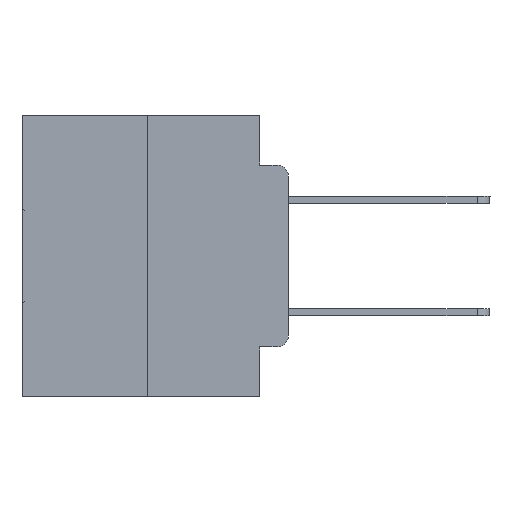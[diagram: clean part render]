
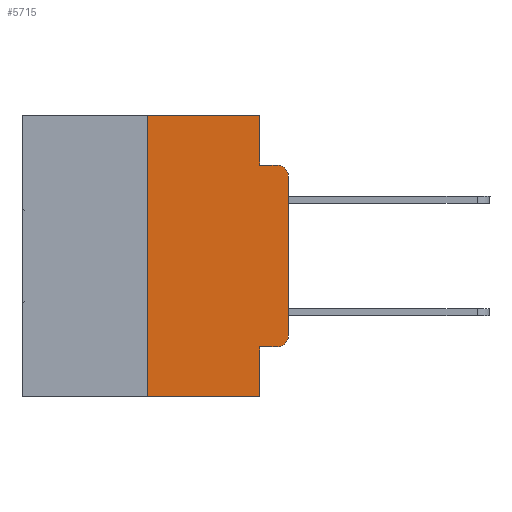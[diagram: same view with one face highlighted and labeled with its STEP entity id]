
A CAD part, left-side view. The second image highlights one B-rep face of the part: STEP entity #5715.
In plain terms, the highlighted planar face has unit normal (-1, 0, 0).
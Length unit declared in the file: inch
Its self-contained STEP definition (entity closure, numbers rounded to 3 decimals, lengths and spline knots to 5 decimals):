
#12 = CARTESIAN_POINT ( 'NONE',  ( 0., 0.473, 0. ) ) ;
#261 = DIRECTION ( 'NONE',  ( 0., 0., -1. ) ) ;
#588 = CARTESIAN_POINT ( 'NONE',  ( 0., 0.02, -0.4115 ) ) ;
#1628 = PLANE ( 'NONE',  #4359 ) ;
#1632 = VERTEX_POINT ( 'NONE', #25571 ) ;
#2724 = VERTEX_POINT ( 'NONE', #16034 ) ;
#2810 = DIRECTION ( 'NONE',  ( -1., 0., 0. ) ) ;
#2978 = VERTEX_POINT ( 'NONE', #13613 ) ;
#3364 = ORIENTED_EDGE ( 'NONE', *, *, #14036, .T. ) ;
#4012 = CARTESIAN_POINT ( 'NONE',  ( 0., 0.473, 0. ) ) ;
#4062 = CARTESIAN_POINT ( 'NONE',  ( 0., 0.051, -0.5 ) ) ;
#4359 = AXIS2_PLACEMENT_3D ( 'NONE', #4012, #8767, #25254 ) ;
#4379 = VECTOR ( 'NONE', #29222, 39.37008 ) ;
#4464 = CARTESIAN_POINT ( 'NONE',  ( 0., 0.051, -0.0885 ) ) ;
#4652 = LINE ( 'NONE', #28440, #22053 ) ;
#4831 = ORIENTED_EDGE ( 'NONE', *, *, #28798, .T. ) ;
#5137 = CIRCLE ( 'NONE', #23619, 0.02 ) ;
#5185 = ORIENTED_EDGE ( 'NONE', *, *, #20552, .T. ) ;
#5715 = ADVANCED_FACE ( 'NONE', ( #9387 ), #1628, .F. ) ;
#6418 = VECTOR ( 'NONE', #9989, 39.37008 ) ;
#7110 = CARTESIAN_POINT ( 'NONE',  ( 0., 0.051, 0. ) ) ;
#7713 = LINE ( 'NONE', #4464, #18872 ) ;
#7816 = EDGE_CURVE ( 'NONE', #29315, #2978, #10740, .T. ) ;
#8767 = DIRECTION ( 'NONE',  ( 1., 0., 0. ) ) ;
#8887 = CARTESIAN_POINT ( 'NONE',  ( 0., 0.02, -0.0885 ) ) ;
#9387 = FACE_OUTER_BOUND ( 'NONE', #10035, .T. ) ;
#9423 = EDGE_CURVE ( 'NONE', #18129, #1632, #4652, .T. ) ;
#9897 = EDGE_CURVE ( 'NONE', #2978, #18129, #11405, .T. ) ;
#9989 = DIRECTION ( 'NONE',  ( 0., -1., 0. ) ) ;
#10035 = EDGE_LOOP ( 'NONE', ( #22578, #5185, #17795, #25488, #26896, #21500, #3364, #22965, #4831, #17447 ) ) ;
#10661 = VECTOR ( 'NONE', #25966, 39.37008 ) ;
#10735 = CARTESIAN_POINT ( 'NONE',  ( 0., 0.02, -0.1085 ) ) ;
#10740 = LINE ( 'NONE', #12974, #4379 ) ;
#10758 = CARTESIAN_POINT ( 'NONE',  ( 0., 0., 0. ) ) ;
#10929 = VERTEX_POINT ( 'NONE', #4062 ) ;
#11058 = EDGE_CURVE ( 'NONE', #1632, #17957, #7713, .T. ) ;
#11405 = LINE ( 'NONE', #12, #10661 ) ;
#12974 = CARTESIAN_POINT ( 'NONE',  ( 0., 0.25, 0. ) ) ;
#13109 = DIRECTION ( 'NONE',  ( 0., 0., -1. ) ) ;
#13494 = LINE ( 'NONE', #26385, #6418 ) ;
#13613 = CARTESIAN_POINT ( 'NONE',  ( 0., 0.25, 0. ) ) ;
#14036 = EDGE_CURVE ( 'NONE', #29315, #10929, #13494, .T. ) ;
#14977 = VECTOR ( 'NONE', #18549, 39.37008 ) ;
#15863 = LINE ( 'NONE', #20847, #26819 ) ;
#16034 = CARTESIAN_POINT ( 'NONE',  ( 0., 0., -0.1085 ) ) ;
#16276 = DIRECTION ( 'NONE',  ( 0., -1., 0. ) ) ;
#17002 = CARTESIAN_POINT ( 'NONE',  ( 0., 0.02, -0.3915 ) ) ;
#17447 = ORIENTED_EDGE ( 'NONE', *, *, #27271, .T. ) ;
#17795 = ORIENTED_EDGE ( 'NONE', *, *, #11058, .F. ) ;
#17957 = VERTEX_POINT ( 'NONE', #8887 ) ;
#18129 = VERTEX_POINT ( 'NONE', #7110 ) ;
#18549 = DIRECTION ( 'NONE',  ( 0., 0., -1. ) ) ;
#18872 = VECTOR ( 'NONE', #16276, 39.37008 ) ;
#19415 = DIRECTION ( 'NONE',  ( 0., 0., -1. ) ) ;
#19728 = CARTESIAN_POINT ( 'NONE',  ( 0., 0., -0.3915 ) ) ;
#19890 = VECTOR ( 'NONE', #24923, 39.37008 ) ;
#20300 = CARTESIAN_POINT ( 'NONE',  ( 0., 0.25, -0.5 ) ) ;
#20552 = EDGE_CURVE ( 'NONE', #2724, #17957, #5137, .T. ) ;
#20611 = LINE ( 'NONE', #10758, #19890 ) ;
#20847 = CARTESIAN_POINT ( 'NONE',  ( 0., 0.051, -0.4115 ) ) ;
#21500 = ORIENTED_EDGE ( 'NONE', *, *, #7816, .F. ) ;
#22053 = VECTOR ( 'NONE', #261, 39.37008 ) ;
#22104 = EDGE_CURVE ( 'NONE', #22651, #2724, #20611, .T. ) ;
#22578 = ORIENTED_EDGE ( 'NONE', *, *, #22104, .T. ) ;
#22651 = VERTEX_POINT ( 'NONE', #19728 ) ;
#22965 = ORIENTED_EDGE ( 'NONE', *, *, #30329, .F. ) ;
#23185 = DIRECTION ( 'NONE',  ( 0., -1., 0. ) ) ;
#23619 = AXIS2_PLACEMENT_3D ( 'NONE', #10735, #27066, #13109 ) ;
#24151 = VERTEX_POINT ( 'NONE', #27874 ) ;
#24923 = DIRECTION ( 'NONE',  ( 0., 0., 1. ) ) ;
#25254 = DIRECTION ( 'NONE',  ( 0., 0., -1. ) ) ;
#25488 = ORIENTED_EDGE ( 'NONE', *, *, #9423, .F. ) ;
#25571 = CARTESIAN_POINT ( 'NONE',  ( 0., 0.051, -0.0885 ) ) ;
#25966 = DIRECTION ( 'NONE',  ( 0., -1., 0. ) ) ;
#26385 = CARTESIAN_POINT ( 'NONE',  ( 0., 0.473, -0.5 ) ) ;
#26819 = VECTOR ( 'NONE', #23185, 39.37008 ) ;
#26896 = ORIENTED_EDGE ( 'NONE', *, *, #9897, .F. ) ;
#27066 = DIRECTION ( 'NONE',  ( -1., 0., 0. ) ) ;
#27271 = EDGE_CURVE ( 'NONE', #29099, #22651, #27963, .T. ) ;
#27874 = CARTESIAN_POINT ( 'NONE',  ( 0., 0.051, -0.4115 ) ) ;
#27963 = CIRCLE ( 'NONE', #29996, 0.02 ) ;
#28440 = CARTESIAN_POINT ( 'NONE',  ( 0., 0.051, 0. ) ) ;
#28762 = LINE ( 'NONE', #30034, #14977 ) ;
#28798 = EDGE_CURVE ( 'NONE', #24151, #29099, #15863, .T. ) ;
#29099 = VERTEX_POINT ( 'NONE', #588 ) ;
#29222 = DIRECTION ( 'NONE',  ( 0., 0., 1. ) ) ;
#29315 = VERTEX_POINT ( 'NONE', #20300 ) ;
#29996 = AXIS2_PLACEMENT_3D ( 'NONE', #17002, #2810, #19415 ) ;
#30034 = CARTESIAN_POINT ( 'NONE',  ( 0., 0.051, 0. ) ) ;
#30329 = EDGE_CURVE ( 'NONE', #24151, #10929, #28762, .T. ) ;
